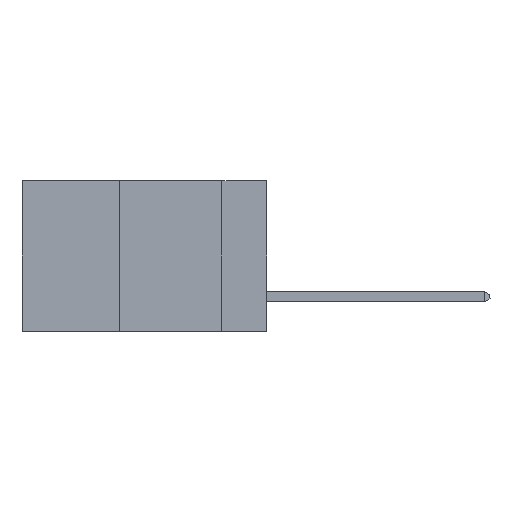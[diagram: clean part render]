
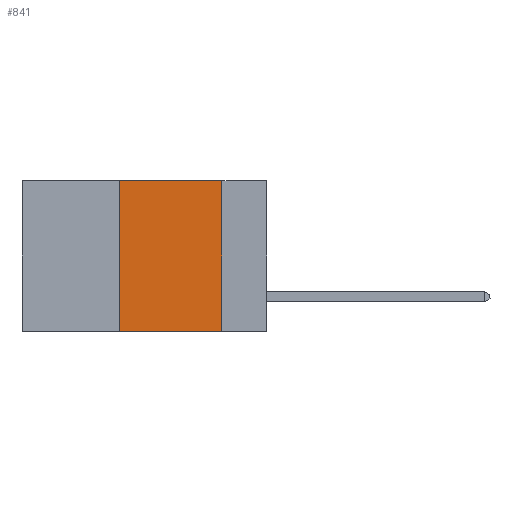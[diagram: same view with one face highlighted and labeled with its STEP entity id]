
A CAD part, left-side view. The second image highlights one B-rep face of the part: STEP entity #841.
In plain terms, the highlighted planar face has unit normal (-1, 0, 0).
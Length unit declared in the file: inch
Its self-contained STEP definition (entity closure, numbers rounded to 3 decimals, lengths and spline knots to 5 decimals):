
#101 = CARTESIAN_POINT ( 'NONE',  ( 0., 0.36, -0.37 ) ) ;
#300 = ORIENTED_EDGE ( 'NONE', *, *, #11532, .F. ) ;
#464 = ORIENTED_EDGE ( 'NONE', *, *, #2325, .F. ) ;
#680 = ORIENTED_EDGE ( 'NONE', *, *, #10753, .F. ) ;
#841 = ADVANCED_FACE ( 'NONE', ( #14667 ), #15494, .F. ) ;
#1015 = CARTESIAN_POINT ( 'NONE',  ( 0., 0.36, 0. ) ) ;
#1109 = EDGE_LOOP ( 'NONE', ( #300, #464, #680, #2195 ) ) ;
#1264 = DIRECTION ( 'NONE',  ( 0., 0., 1. ) ) ;
#1397 = VERTEX_POINT ( 'NONE', #1015 ) ;
#2195 = ORIENTED_EDGE ( 'NONE', *, *, #9943, .T. ) ;
#2325 = EDGE_CURVE ( 'NONE', #1397, #11619, #9072, .T. ) ;
#2745 = DIRECTION ( 'NONE',  ( 0., -1., 0. ) ) ;
#3594 = VECTOR ( 'NONE', #4201, 39.37008 ) ;
#4201 = DIRECTION ( 'NONE',  ( 0., 0., -1. ) ) ;
#4939 = AXIS2_PLACEMENT_3D ( 'NONE', #15069, #14554, #14866 ) ;
#6058 = LINE ( 'NONE', #8897, #9719 ) ;
#7043 = VERTEX_POINT ( 'NONE', #13027 ) ;
#7108 = CARTESIAN_POINT ( 'NONE',  ( 0., 0.6, 0. ) ) ;
#7167 = DIRECTION ( 'NONE',  ( 0., -1., 0. ) ) ;
#7453 = VECTOR ( 'NONE', #2745, 39.37008 ) ;
#8897 = CARTESIAN_POINT ( 'NONE',  ( 0., 0.36, 0. ) ) ;
#9072 = LINE ( 'NONE', #7108, #11889 ) ;
#9210 = CARTESIAN_POINT ( 'NONE',  ( 0., 0.11, 0. ) ) ;
#9719 = VECTOR ( 'NONE', #1264, 39.37008 ) ;
#9943 = EDGE_CURVE ( 'NONE', #11400, #7043, #10686, .T. ) ;
#10686 = LINE ( 'NONE', #13668, #7453 ) ;
#10753 = EDGE_CURVE ( 'NONE', #11400, #1397, #6058, .T. ) ;
#11400 = VERTEX_POINT ( 'NONE', #101 ) ;
#11532 = EDGE_CURVE ( 'NONE', #11619, #7043, #12982, .T. ) ;
#11619 = VERTEX_POINT ( 'NONE', #11719 ) ;
#11719 = CARTESIAN_POINT ( 'NONE',  ( 0., 0.11, 0. ) ) ;
#11889 = VECTOR ( 'NONE', #7167, 39.37008 ) ;
#12982 = LINE ( 'NONE', #9210, #3594 ) ;
#13027 = CARTESIAN_POINT ( 'NONE',  ( 0., 0.11, -0.37 ) ) ;
#13668 = CARTESIAN_POINT ( 'NONE',  ( 0., 0.6, -0.37 ) ) ;
#14554 = DIRECTION ( 'NONE',  ( 1., 0., 0. ) ) ;
#14667 = FACE_OUTER_BOUND ( 'NONE', #1109, .T. ) ;
#14866 = DIRECTION ( 'NONE',  ( 0., 0., -1. ) ) ;
#15069 = CARTESIAN_POINT ( 'NONE',  ( 0., 0.6, 0. ) ) ;
#15494 = PLANE ( 'NONE',  #4939 ) ;
